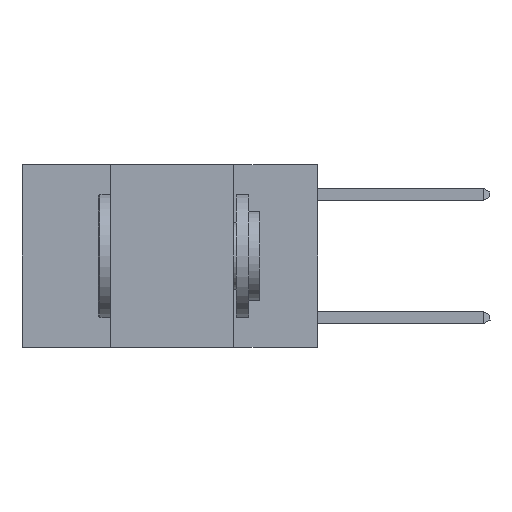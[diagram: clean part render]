
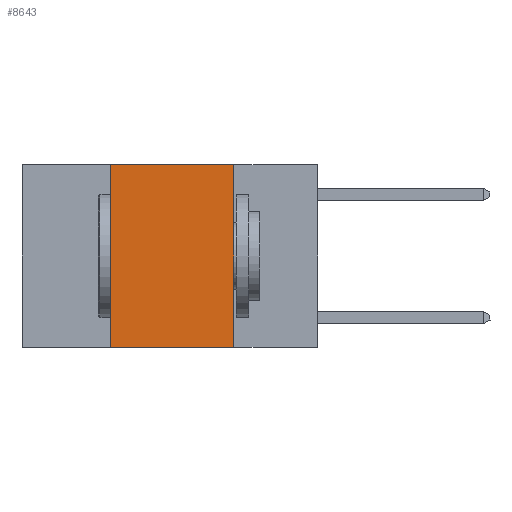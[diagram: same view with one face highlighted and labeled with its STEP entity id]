
A CAD part, left-side view. The second image highlights one B-rep face of the part: STEP entity #8643.
In plain terms, the highlighted planar face has unit normal (-1, 0, 0).
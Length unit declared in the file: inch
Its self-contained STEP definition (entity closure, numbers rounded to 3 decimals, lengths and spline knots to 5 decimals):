
#239 = CARTESIAN_POINT ( 'NONE',  ( 0., 0.42, 0. ) ) ;
#386 = CARTESIAN_POINT ( 'NONE',  ( 0., 0.17, 0. ) ) ;
#562 = VERTEX_POINT ( 'NONE', #386 ) ;
#1191 = CARTESIAN_POINT ( 'NONE',  ( 0., 0.42, 0. ) ) ;
#1538 = DIRECTION ( 'NONE',  ( 0., 0., -1. ) ) ;
#1848 = CARTESIAN_POINT ( 'NONE',  ( 0., 0.42, -0.37 ) ) ;
#2364 = EDGE_CURVE ( 'NONE', #562, #12578, #22721, .T. ) ;
#2725 = FACE_OUTER_BOUND ( 'NONE', #19685, .T. ) ;
#3202 = ORIENTED_EDGE ( 'NONE', *, *, #3595, .F. ) ;
#3595 = EDGE_CURVE ( 'NONE', #14478, #19116, #27731, .T. ) ;
#4590 = VECTOR ( 'NONE', #25164, 39.37008 ) ;
#5679 = DIRECTION ( 'NONE',  ( 0., 0., 1. ) ) ;
#7440 = LINE ( 'NONE', #23036, #19024 ) ;
#7669 = ORIENTED_EDGE ( 'NONE', *, *, #12934, .F. ) ;
#7796 = CARTESIAN_POINT ( 'NONE',  ( 0., 0.6, 0. ) ) ;
#8469 = AXIS2_PLACEMENT_3D ( 'NONE', #27638, #14687, #1538 ) ;
#8643 = ADVANCED_FACE ( 'NONE', ( #2725 ), #21148, .F. ) ;
#10305 = EDGE_CURVE ( 'NONE', #14478, #12578, #7440, .T. ) ;
#10449 = VECTOR ( 'NONE', #5679, 39.37008 ) ;
#12488 = CARTESIAN_POINT ( 'NONE',  ( 0., 0.17, 0. ) ) ;
#12578 = VERTEX_POINT ( 'NONE', #26123 ) ;
#12934 = EDGE_CURVE ( 'NONE', #19116, #562, #27679, .T. ) ;
#14478 = VERTEX_POINT ( 'NONE', #1848 ) ;
#14687 = DIRECTION ( 'NONE',  ( 1., 0., 0. ) ) ;
#16193 = ORIENTED_EDGE ( 'NONE', *, *, #10305, .T. ) ;
#17619 = VECTOR ( 'NONE', #27632, 39.37008 ) ;
#19024 = VECTOR ( 'NONE', #25189, 39.37008 ) ;
#19116 = VERTEX_POINT ( 'NONE', #239 ) ;
#19685 = EDGE_LOOP ( 'NONE', ( #23641, #7669, #3202, #16193 ) ) ;
#21148 = PLANE ( 'NONE',  #8469 ) ;
#22721 = LINE ( 'NONE', #12488, #17619 ) ;
#23036 = CARTESIAN_POINT ( 'NONE',  ( 0., 0.6, -0.37 ) ) ;
#23641 = ORIENTED_EDGE ( 'NONE', *, *, #2364, .F. ) ;
#25164 = DIRECTION ( 'NONE',  ( 0., -1., 0. ) ) ;
#25189 = DIRECTION ( 'NONE',  ( 0., -1., 0. ) ) ;
#26123 = CARTESIAN_POINT ( 'NONE',  ( 0., 0.17, -0.37 ) ) ;
#27632 = DIRECTION ( 'NONE',  ( 0., 0., -1. ) ) ;
#27638 = CARTESIAN_POINT ( 'NONE',  ( 0., 0.6, 0. ) ) ;
#27679 = LINE ( 'NONE', #7796, #4590 ) ;
#27731 = LINE ( 'NONE', #1191, #10449 ) ;
